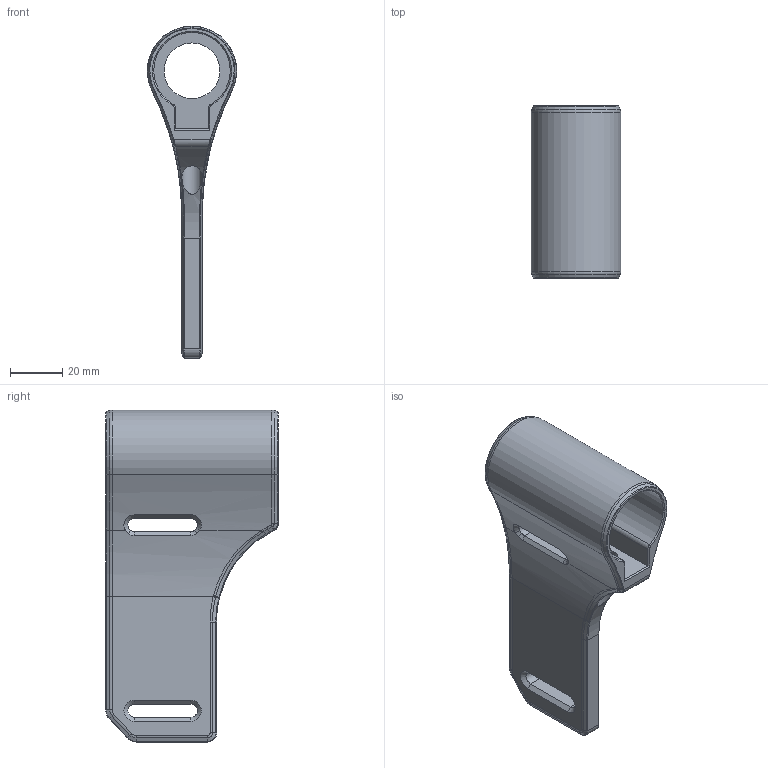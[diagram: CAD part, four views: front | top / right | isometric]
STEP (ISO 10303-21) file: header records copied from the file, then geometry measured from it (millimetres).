
FILE_DESCRIPTION(/* description */ (''),/* implementation_level */ '2;1');
FILE_NAME(/* name */ 'Minimalist Pistol Brace (MPB).step',/* time_stamp */ '2021-04-17T01:45:50-04:00',/* author */ (''),/* organization */ (''),/* preprocessor_version */ 'ST-DEVELOPER v18.1',/* originating_system */ 'Autodesk Translation Framework v10.6.0.1341',/* authorisation */ '');
FILE_SCHEMA (('AUTOMOTIVE_DESIGN { 1 0 10303 214 3 1 1 }'));
Length unit declared in the file: millimetre
Products named in the file (1): Minimalist Pistol Brace (MPB)
Bounding box: 34.37 x 66.31 x 127.5 mm (x, y, z)
Volume: 55593.3 mm3; surface area: 25999.9 mm2
Topology: 1 solids, 1 shells, 196 faces, 451 edges, 255 vertices
Faces by surface type: bspline 76, cone 40, plane 38, cylinder 28, torus 14
Full cylindrical faces by diameter (mm): 7.75 x1, 21.4 x1
Entity records: 7137 total; most frequent: CARTESIAN_POINT 3092, ORIENTED_EDGE 902, DIRECTION 701, EDGE_CURVE 451, VERTEX_POINT 255, AXIS2_PLACEMENT_3D 254, EDGE_LOOP 202, FACE_OUTER_BOUND 196
